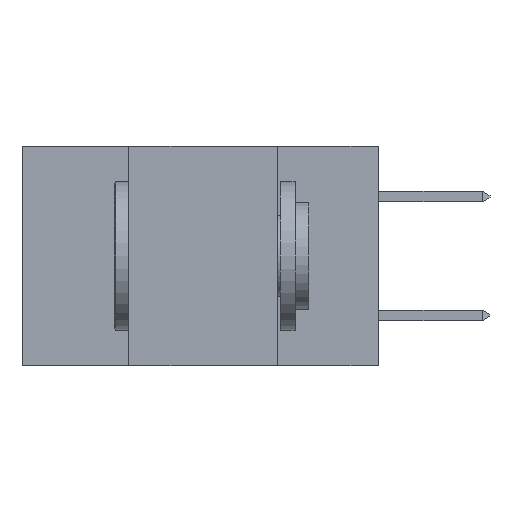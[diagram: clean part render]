
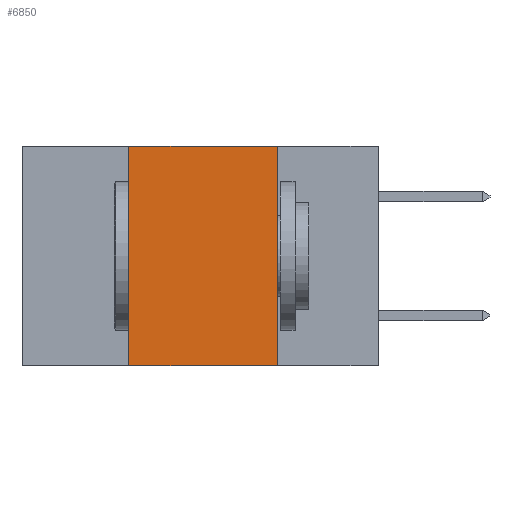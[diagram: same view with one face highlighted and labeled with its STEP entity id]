
A CAD part, left-side view. The second image highlights one B-rep face of the part: STEP entity #6850.
In plain terms, the highlighted planar face has unit normal (-1, 0, 0).
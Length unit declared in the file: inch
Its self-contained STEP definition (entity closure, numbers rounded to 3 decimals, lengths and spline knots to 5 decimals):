
#119 = ORIENTED_EDGE ( 'NONE', *, *, #10428, .F. ) ;
#1458 = CARTESIAN_POINT ( 'NONE',  ( 0., 0.6, 0. ) ) ;
#2249 = ORIENTED_EDGE ( 'NONE', *, *, #16743, .F. ) ;
#2419 = VERTEX_POINT ( 'NONE', #17127 ) ;
#2785 = VECTOR ( 'NONE', #11519, 39.37008 ) ;
#6850 = ADVANCED_FACE ( 'NONE', ( #13099 ), #9225, .F. ) ;
#8646 = CARTESIAN_POINT ( 'NONE',  ( 0., 0.42, 0. ) ) ;
#9225 = PLANE ( 'NONE',  #24454 ) ;
#9515 = EDGE_CURVE ( 'NONE', #20755, #16055, #12597, .T. ) ;
#10428 = EDGE_CURVE ( 'NONE', #16055, #22746, #22497, .T. ) ;
#11519 = DIRECTION ( 'NONE',  ( 0., -1., 0. ) ) ;
#11701 = DIRECTION ( 'NONE',  ( 0., 0., -1. ) ) ;
#12597 = LINE ( 'NONE', #13172, #30793 ) ;
#13099 = FACE_OUTER_BOUND ( 'NONE', #15008, .T. ) ;
#13172 = CARTESIAN_POINT ( 'NONE',  ( 0., 0.42, 0. ) ) ;
#15008 = EDGE_LOOP ( 'NONE', ( #2249, #119, #28118, #31215 ) ) ;
#16055 = VERTEX_POINT ( 'NONE', #8646 ) ;
#16743 = EDGE_CURVE ( 'NONE', #22746, #2419, #24843, .T. ) ;
#17127 = CARTESIAN_POINT ( 'NONE',  ( 0., 0.17, -0.37 ) ) ;
#18280 = VECTOR ( 'NONE', #25867, 39.37008 ) ;
#18830 = CARTESIAN_POINT ( 'NONE',  ( 0., 0.42, -0.37 ) ) ;
#19438 = EDGE_CURVE ( 'NONE', #20755, #2419, #20969, .T. ) ;
#20214 = VECTOR ( 'NONE', #31054, 39.37008 ) ;
#20258 = CARTESIAN_POINT ( 'NONE',  ( 0., 0.17, 0. ) ) ;
#20591 = DIRECTION ( 'NONE',  ( 0., 0., 1. ) ) ;
#20755 = VERTEX_POINT ( 'NONE', #18830 ) ;
#20969 = LINE ( 'NONE', #21131, #20214 ) ;
#21131 = CARTESIAN_POINT ( 'NONE',  ( 0., 0.6, -0.37 ) ) ;
#22497 = LINE ( 'NONE', #1458, #2785 ) ;
#22746 = VERTEX_POINT ( 'NONE', #20258 ) ;
#24454 = AXIS2_PLACEMENT_3D ( 'NONE', #28917, #26523, #11701 ) ;
#24843 = LINE ( 'NONE', #30762, #18280 ) ;
#25867 = DIRECTION ( 'NONE',  ( 0., 0., -1. ) ) ;
#26523 = DIRECTION ( 'NONE',  ( 1., 0., 0. ) ) ;
#28118 = ORIENTED_EDGE ( 'NONE', *, *, #9515, .F. ) ;
#28917 = CARTESIAN_POINT ( 'NONE',  ( 0., 0.6, 0. ) ) ;
#30762 = CARTESIAN_POINT ( 'NONE',  ( 0., 0.17, 0. ) ) ;
#30793 = VECTOR ( 'NONE', #20591, 39.37008 ) ;
#31054 = DIRECTION ( 'NONE',  ( 0., -1., 0. ) ) ;
#31215 = ORIENTED_EDGE ( 'NONE', *, *, #19438, .T. ) ;
